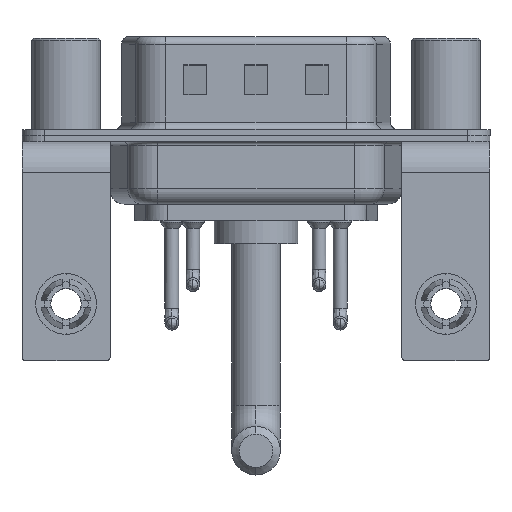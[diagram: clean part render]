
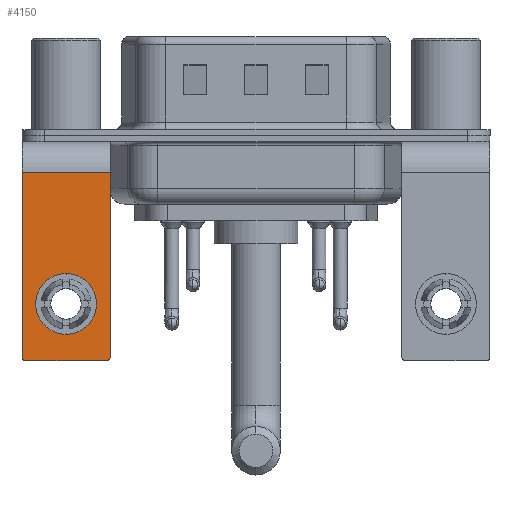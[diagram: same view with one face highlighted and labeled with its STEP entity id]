
A CAD part, front view. The second image highlights one B-rep face of the part: STEP entity #4150.
In plain terms, the highlighted planar face has unit normal (0, -1, 0).
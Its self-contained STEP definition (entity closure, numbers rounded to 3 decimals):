
#150 = AXIS2_PLACEMENT_3D ( 'NONE', #10489, #5386, #19861 ) ;
#806 = CARTESIAN_POINT ( 'NONE',  ( -2.9, -6.25, -14.55 ) ) ;
#951 = DIRECTION ( 'NONE',  ( 0., 1., 0. ) ) ;
#2016 = CARTESIAN_POINT ( 'NONE',  ( 2.9, -6.25, -2.4 ) ) ;
#2201 = EDGE_CURVE ( 'NONE', #14792, #21121, #11139, .T. ) ;
#2214 = VECTOR ( 'NONE', #4615, 1000. ) ;
#2340 = CARTESIAN_POINT ( 'NONE',  ( 0., -6.25, -11.07 ) ) ;
#2513 = ORIENTED_EDGE ( 'NONE', *, *, #19052, .T. ) ;
#2602 = DIRECTION ( 'NONE',  ( 0., 0., 1. ) ) ;
#2650 = VERTEX_POINT ( 'NONE', #806 ) ;
#2872 = ORIENTED_EDGE ( 'NONE', *, *, #12946, .F. ) ;
#3347 = DIRECTION ( 'NONE',  ( 0., -1., 0. ) ) ;
#3432 = FACE_OUTER_BOUND ( 'NONE', #18622, .T. ) ;
#3459 = ORIENTED_EDGE ( 'NONE', *, *, #11155, .F. ) ;
#3477 = CARTESIAN_POINT ( 'NONE',  ( 0., -6.25, -9.07 ) ) ;
#3532 = VERTEX_POINT ( 'NONE', #14812 ) ;
#3601 = CARTESIAN_POINT ( 'NONE',  ( 2.9, -6.25, -2.4 ) ) ;
#4150 = ADVANCED_FACE ( 'NONE', ( #6761, #3432 ), #8621, .F. ) ;
#4483 = DIRECTION ( 'NONE',  ( 0., -1., 0. ) ) ;
#4615 = DIRECTION ( 'NONE',  ( 0., 0., -1. ) ) ;
#4900 = CARTESIAN_POINT ( 'NONE',  ( 0., -6.25, -11.07 ) ) ;
#5386 = DIRECTION ( 'NONE',  ( 0., 1., 0. ) ) ;
#5637 = ORIENTED_EDGE ( 'NONE', *, *, #2201, .T. ) ;
#5949 = AXIS2_PLACEMENT_3D ( 'NONE', #2340, #951, #21657 ) ;
#6761 = FACE_BOUND ( 'NONE', #18445, .T. ) ;
#6946 = VERTEX_POINT ( 'NONE', #15122 ) ;
#8080 = CARTESIAN_POINT ( 'NONE',  ( 0., -6.25, -13.07 ) ) ;
#8129 = CIRCLE ( 'NONE', #18872, 2. ) ;
#8620 = VECTOR ( 'NONE', #11413, 1000. ) ;
#8621 = PLANE ( 'NONE',  #150 ) ;
#8663 = ORIENTED_EDGE ( 'NONE', *, *, #18791, .T. ) ;
#9446 = CIRCLE ( 'NONE', #15348, 0.25 ) ;
#9476 = VERTEX_POINT ( 'NONE', #12496 ) ;
#9564 = VECTOR ( 'NONE', #14327, 1000. ) ;
#9761 = ORIENTED_EDGE ( 'NONE', *, *, #15220, .T. ) ;
#10489 = CARTESIAN_POINT ( 'NONE',  ( 2.9, -6.25, -2.4 ) ) ;
#11088 = LINE ( 'NONE', #21626, #9564 ) ;
#11139 = CIRCLE ( 'NONE', #5949, 2. ) ;
#11155 = EDGE_CURVE ( 'NONE', #3532, #9476, #11088, .T. ) ;
#11311 = CARTESIAN_POINT ( 'NONE',  ( 2.65, -6.25, -14.55 ) ) ;
#11413 = DIRECTION ( 'NONE',  ( 0., 0., -1. ) ) ;
#11952 = DIRECTION ( 'NONE',  ( 0., 1., 0. ) ) ;
#12117 = DIRECTION ( 'NONE',  ( 0., 0., 1. ) ) ;
#12496 = CARTESIAN_POINT ( 'NONE',  ( -2.65, -6.25, -14.8 ) ) ;
#12602 = ORIENTED_EDGE ( 'NONE', *, *, #14797, .T. ) ;
#12946 = EDGE_CURVE ( 'NONE', #14523, #15444, #16621, .T. ) ;
#14327 = DIRECTION ( 'NONE',  ( -1., 0., 0. ) ) ;
#14444 = EDGE_CURVE ( 'NONE', #6946, #2650, #16879, .T. ) ;
#14523 = VERTEX_POINT ( 'NONE', #21525 ) ;
#14792 = VERTEX_POINT ( 'NONE', #8080 ) ;
#14797 = EDGE_CURVE ( 'NONE', #2650, #9476, #9446, .T. ) ;
#14812 = CARTESIAN_POINT ( 'NONE',  ( 2.65, -6.25, -14.8 ) ) ;
#15122 = CARTESIAN_POINT ( 'NONE',  ( -2.9, -6.25, -2.4 ) ) ;
#15130 = CARTESIAN_POINT ( 'NONE',  ( -2.9, -6.25, -2.4 ) ) ;
#15220 = EDGE_CURVE ( 'NONE', #3532, #15444, #16195, .T. ) ;
#15348 = AXIS2_PLACEMENT_3D ( 'NONE', #19089, #3347, #12117 ) ;
#15444 = VERTEX_POINT ( 'NONE', #21255 ) ;
#16195 = CIRCLE ( 'NONE', #19549, 0.25 ) ;
#16621 = LINE ( 'NONE', #3601, #8620 ) ;
#16879 = LINE ( 'NONE', #15130, #2214 ) ;
#18144 = VECTOR ( 'NONE', #19946, 1000. ) ;
#18445 = EDGE_LOOP ( 'NONE', ( #5637, #8663 ) ) ;
#18622 = EDGE_LOOP ( 'NONE', ( #21752, #12602, #3459, #9761, #2872, #2513 ) ) ;
#18791 = EDGE_CURVE ( 'NONE', #21121, #14792, #8129, .T. ) ;
#18872 = AXIS2_PLACEMENT_3D ( 'NONE', #4900, #11952, #2602 ) ;
#19052 = EDGE_CURVE ( 'NONE', #14523, #6946, #21447, .T. ) ;
#19089 = CARTESIAN_POINT ( 'NONE',  ( -2.65, -6.25, -14.55 ) ) ;
#19549 = AXIS2_PLACEMENT_3D ( 'NONE', #11311, #4483, #21951 ) ;
#19861 = DIRECTION ( 'NONE',  ( 0., 0., 1. ) ) ;
#19946 = DIRECTION ( 'NONE',  ( -1., 0., 0. ) ) ;
#21121 = VERTEX_POINT ( 'NONE', #3477 ) ;
#21255 = CARTESIAN_POINT ( 'NONE',  ( 2.9, -6.25, -14.55 ) ) ;
#21447 = LINE ( 'NONE', #2016, #18144 ) ;
#21525 = CARTESIAN_POINT ( 'NONE',  ( 2.9, -6.25, -2.4 ) ) ;
#21626 = CARTESIAN_POINT ( 'NONE',  ( 2.9, -6.25, -14.8 ) ) ;
#21657 = DIRECTION ( 'NONE',  ( 0., 0., 1. ) ) ;
#21752 = ORIENTED_EDGE ( 'NONE', *, *, #14444, .T. ) ;
#21951 = DIRECTION ( 'NONE',  ( 0., 0., 1. ) ) ;
